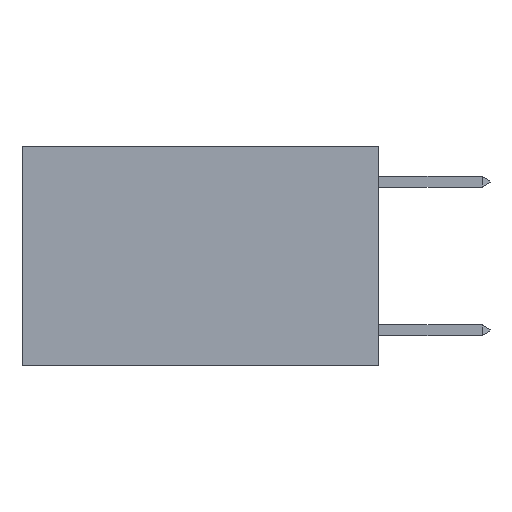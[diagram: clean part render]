
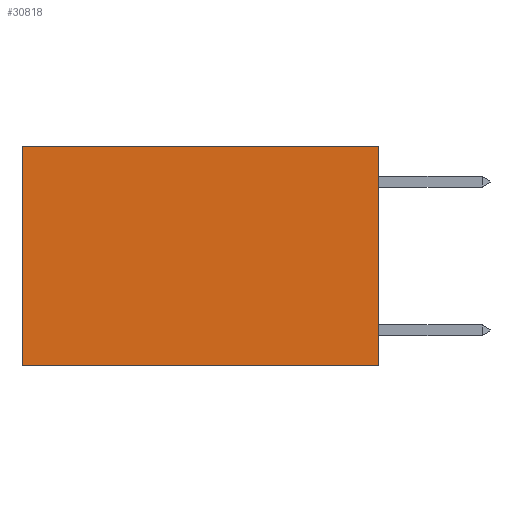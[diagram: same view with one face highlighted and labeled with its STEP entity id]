
A CAD part, left-side view. The second image highlights one B-rep face of the part: STEP entity #30818.
In plain terms, the highlighted planar face has unit normal (-1, 0, 0).
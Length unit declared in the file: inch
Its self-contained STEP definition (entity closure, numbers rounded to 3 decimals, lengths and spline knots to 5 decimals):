
#201 = AXIS2_PLACEMENT_3D ( 'NONE', #2732, #503, #21708 ) ;
#351 = CARTESIAN_POINT ( 'NONE',  ( 0.2625, 0.6, 0. ) ) ;
#503 = DIRECTION ( 'NONE',  ( 1., 0., 0. ) ) ;
#1673 = CARTESIAN_POINT ( 'NONE',  ( 0.2625, 0., -0.37 ) ) ;
#1949 = LINE ( 'NONE', #24581, #24330 ) ;
#2732 = CARTESIAN_POINT ( 'NONE',  ( 0.2625, 0., 0. ) ) ;
#3638 = VECTOR ( 'NONE', #30265, 39.37008 ) ;
#3750 = LINE ( 'NONE', #9242, #11963 ) ;
#4103 = EDGE_CURVE ( 'NONE', #22401, #18142, #9991, .T. ) ;
#6339 = CARTESIAN_POINT ( 'NONE',  ( 0.2625, 0., 0. ) ) ;
#7837 = EDGE_LOOP ( 'NONE', ( #21928, #26533, #28274, #18774 ) ) ;
#8130 = DIRECTION ( 'NONE',  ( 0., 1., 0. ) ) ;
#9242 = CARTESIAN_POINT ( 'NONE',  ( 0.2625, 0., 0. ) ) ;
#9991 = LINE ( 'NONE', #6339, #3638 ) ;
#11770 = FACE_OUTER_BOUND ( 'NONE', #7837, .T. ) ;
#11781 = CARTESIAN_POINT ( 'NONE',  ( 0.2625, 0., 0. ) ) ;
#11963 = VECTOR ( 'NONE', #23590, 39.37008 ) ;
#12278 = DIRECTION ( 'NONE',  ( 0., 0., -1. ) ) ;
#13909 = CARTESIAN_POINT ( 'NONE',  ( 0.2625, 0.6, 0. ) ) ;
#16307 = EDGE_CURVE ( 'NONE', #22401, #25877, #3750, .T. ) ;
#16621 = VECTOR ( 'NONE', #12278, 39.37008 ) ;
#18142 = VERTEX_POINT ( 'NONE', #1673 ) ;
#18774 = ORIENTED_EDGE ( 'NONE', *, *, #16307, .T. ) ;
#18930 = EDGE_CURVE ( 'NONE', #25877, #20577, #29633, .T. ) ;
#20577 = VERTEX_POINT ( 'NONE', #26840 ) ;
#20583 = EDGE_CURVE ( 'NONE', #18142, #20577, #1949, .T. ) ;
#21708 = DIRECTION ( 'NONE',  ( 0., 0., -1. ) ) ;
#21928 = ORIENTED_EDGE ( 'NONE', *, *, #18930, .T. ) ;
#22401 = VERTEX_POINT ( 'NONE', #11781 ) ;
#23590 = DIRECTION ( 'NONE',  ( 0., 1., 0. ) ) ;
#24082 = PLANE ( 'NONE',  #201 ) ;
#24330 = VECTOR ( 'NONE', #8130, 39.37008 ) ;
#24581 = CARTESIAN_POINT ( 'NONE',  ( 0.2625, 0., -0.37 ) ) ;
#25877 = VERTEX_POINT ( 'NONE', #13909 ) ;
#26533 = ORIENTED_EDGE ( 'NONE', *, *, #20583, .F. ) ;
#26840 = CARTESIAN_POINT ( 'NONE',  ( 0.2625, 0.6, -0.37 ) ) ;
#28274 = ORIENTED_EDGE ( 'NONE', *, *, #4103, .F. ) ;
#29633 = LINE ( 'NONE', #351, #16621 ) ;
#30265 = DIRECTION ( 'NONE',  ( 0., 0., -1. ) ) ;
#30818 = ADVANCED_FACE ( 'NONE', ( #11770 ), #24082, .F. ) ;
